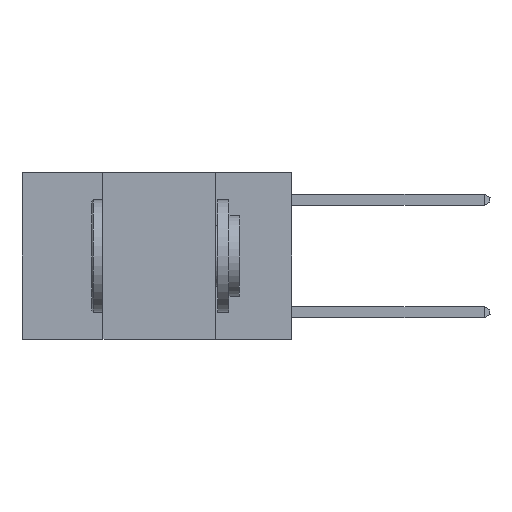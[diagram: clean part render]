
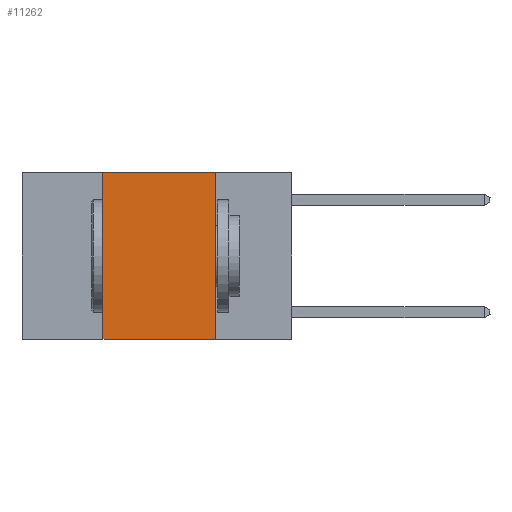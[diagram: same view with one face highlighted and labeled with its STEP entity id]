
A CAD part, left-side view. The second image highlights one B-rep face of the part: STEP entity #11262.
In plain terms, the highlighted planar face has unit normal (-1, 0, 0).
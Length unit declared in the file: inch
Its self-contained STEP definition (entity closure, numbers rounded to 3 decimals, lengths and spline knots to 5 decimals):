
#69 = ORIENTED_EDGE ( 'NONE', *, *, #4070, .F. ) ;
#709 = VERTEX_POINT ( 'NONE', #9901 ) ;
#745 = CARTESIAN_POINT ( 'NONE',  ( 0., 0.17, -0.37 ) ) ;
#1433 = CARTESIAN_POINT ( 'NONE',  ( 0., 0.17, 0. ) ) ;
#1973 = VECTOR ( 'NONE', #4623, 39.37008 ) ;
#2583 = VECTOR ( 'NONE', #5340, 39.37008 ) ;
#2659 = CARTESIAN_POINT ( 'NONE',  ( 0., 0.6, -0.37 ) ) ;
#3394 = CARTESIAN_POINT ( 'NONE',  ( 0., 0.6, 0. ) ) ;
#4070 = EDGE_CURVE ( 'NONE', #8922, #10939, #8316, .T. ) ;
#4269 = EDGE_CURVE ( 'NONE', #709, #10939, #10379, .T. ) ;
#4568 = VECTOR ( 'NONE', #12055, 39.37008 ) ;
#4623 = DIRECTION ( 'NONE',  ( 0., -1., 0. ) ) ;
#5193 = EDGE_LOOP ( 'NONE', ( #69, #8078, #6838, #11602 ) ) ;
#5195 = DIRECTION ( 'NONE',  ( 1., 0., 0. ) ) ;
#5340 = DIRECTION ( 'NONE',  ( 0., 0., -1. ) ) ;
#5346 = CARTESIAN_POINT ( 'NONE',  ( 0., 0.42, 0. ) ) ;
#5622 = EDGE_CURVE ( 'NONE', #709, #7127, #7175, .T. ) ;
#6054 = CARTESIAN_POINT ( 'NONE',  ( 0., 0.42, 0. ) ) ;
#6230 = LINE ( 'NONE', #3394, #4568 ) ;
#6838 = ORIENTED_EDGE ( 'NONE', *, *, #5622, .F. ) ;
#7095 = CARTESIAN_POINT ( 'NONE',  ( 0., 0.6, 0. ) ) ;
#7127 = VERTEX_POINT ( 'NONE', #6054 ) ;
#7146 = DIRECTION ( 'NONE',  ( 0., 0., -1. ) ) ;
#7175 = LINE ( 'NONE', #5346, #8221 ) ;
#7216 = PLANE ( 'NONE',  #12488 ) ;
#8078 = ORIENTED_EDGE ( 'NONE', *, *, #11202, .F. ) ;
#8221 = VECTOR ( 'NONE', #11893, 39.37008 ) ;
#8316 = LINE ( 'NONE', #1433, #2583 ) ;
#8922 = VERTEX_POINT ( 'NONE', #9969 ) ;
#9901 = CARTESIAN_POINT ( 'NONE',  ( 0., 0.42, -0.37 ) ) ;
#9969 = CARTESIAN_POINT ( 'NONE',  ( 0., 0.17, 0. ) ) ;
#10379 = LINE ( 'NONE', #2659, #1973 ) ;
#10939 = VERTEX_POINT ( 'NONE', #745 ) ;
#11202 = EDGE_CURVE ( 'NONE', #7127, #8922, #6230, .T. ) ;
#11262 = ADVANCED_FACE ( 'NONE', ( #11927 ), #7216, .F. ) ;
#11602 = ORIENTED_EDGE ( 'NONE', *, *, #4269, .T. ) ;
#11893 = DIRECTION ( 'NONE',  ( 0., 0., 1. ) ) ;
#11927 = FACE_OUTER_BOUND ( 'NONE', #5193, .T. ) ;
#12055 = DIRECTION ( 'NONE',  ( 0., -1., 0. ) ) ;
#12488 = AXIS2_PLACEMENT_3D ( 'NONE', #7095, #5195, #7146 ) ;
